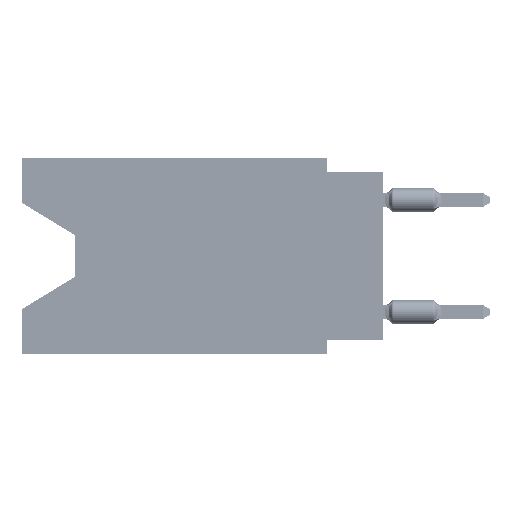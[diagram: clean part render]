
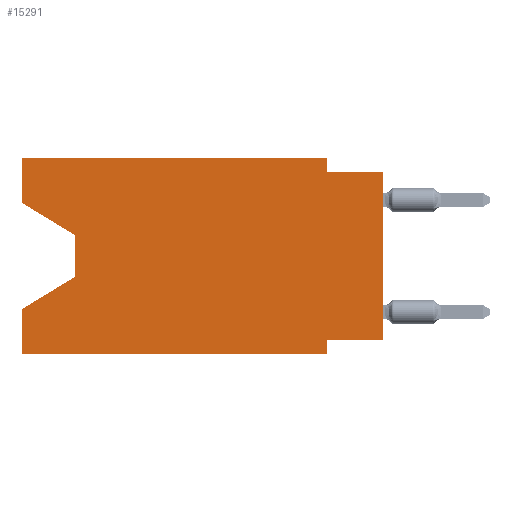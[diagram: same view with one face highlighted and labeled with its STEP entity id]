
A CAD part, left-side view. The second image highlights one B-rep face of the part: STEP entity #15291.
In plain terms, the highlighted planar face has unit normal (-1, 0, 0).
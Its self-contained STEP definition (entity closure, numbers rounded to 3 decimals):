
#107 = CARTESIAN_POINT ( 'NONE',  ( 0., 16.383, 0. ) ) ;
#763 = DIRECTION ( 'NONE',  ( 0., -0.855, -0.519 ) ) ;
#1878 = EDGE_CURVE ( 'NONE', #25673, #46017, #35333, .T. ) ;
#1930 = CARTESIAN_POINT ( 'NONE',  ( 0., 16.383, -2.038 ) ) ;
#2793 = AXIS2_PLACEMENT_3D ( 'NONE', #67931, #42210, #43051 ) ;
#2874 = DIRECTION ( 'NONE',  ( 0., 0., -1. ) ) ;
#2944 = VECTOR ( 'NONE', #48838, 1000. ) ;
#3037 = LINE ( 'NONE', #9887, #2944 ) ;
#4022 = LINE ( 'NONE', #82381, #73340 ) ;
#4577 = ORIENTED_EDGE ( 'NONE', *, *, #26708, .F. ) ;
#4982 = VECTOR ( 'NONE', #763, 1000. ) ;
#5463 = CARTESIAN_POINT ( 'NONE',  ( 0., 13.97, -5.385 ) ) ;
#9887 = CARTESIAN_POINT ( 'NONE',  ( 0., 16.383, 0. ) ) ;
#12253 = CARTESIAN_POINT ( 'NONE',  ( 0., 2.54, -8.255 ) ) ;
#14209 = LINE ( 'NONE', #107, #69110 ) ;
#15291 = ADVANCED_FACE ( 'NONE', ( #48216 ), #36222, .F. ) ;
#15348 = EDGE_CURVE ( 'NONE', #16170, #65032, #21712, .T. ) ;
#16145 = LINE ( 'NONE', #35400, #50735 ) ;
#16170 = VERTEX_POINT ( 'NONE', #39067 ) ;
#16558 = DIRECTION ( 'NONE',  ( 0., -1., 0. ) ) ;
#16648 = VECTOR ( 'NONE', #29829, 1000. ) ;
#17340 = EDGE_CURVE ( 'NONE', #54386, #83672, #40953, .T. ) ;
#19765 = EDGE_CURVE ( 'NONE', #46017, #43239, #67621, .T. ) ;
#20991 = CARTESIAN_POINT ( 'NONE',  ( 0., 16.383, -8.89 ) ) ;
#21712 = LINE ( 'NONE', #22974, #43765 ) ;
#22974 = CARTESIAN_POINT ( 'NONE',  ( 0., 0., -8.255 ) ) ;
#23085 = CARTESIAN_POINT ( 'NONE',  ( 0., 0., -0.635 ) ) ;
#23415 = CARTESIAN_POINT ( 'NONE',  ( 0., 13.97, -3.505 ) ) ;
#25673 = VERTEX_POINT ( 'NONE', #26415 ) ;
#26223 = CARTESIAN_POINT ( 'NONE',  ( 0., 0., 0. ) ) ;
#26322 = VECTOR ( 'NONE', #49864, 1000. ) ;
#26415 = CARTESIAN_POINT ( 'NONE',  ( 0., 2.54, 0. ) ) ;
#26708 = EDGE_CURVE ( 'NONE', #51385, #32108, #3037, .T. ) ;
#26897 = EDGE_CURVE ( 'NONE', #65584, #54386, #36257, .T. ) ;
#27863 = CARTESIAN_POINT ( 'NONE',  ( 0., 16.383, -6.852 ) ) ;
#28916 = CARTESIAN_POINT ( 'NONE',  ( 0., 2.54, 0. ) ) ;
#29567 = ORIENTED_EDGE ( 'NONE', *, *, #56572, .T. ) ;
#29829 = DIRECTION ( 'NONE',  ( 0., 0.855, -0.519 ) ) ;
#30577 = CARTESIAN_POINT ( 'NONE',  ( 0., 2.54, -0.635 ) ) ;
#30886 = CARTESIAN_POINT ( 'NONE',  ( 0., 16.383, 0. ) ) ;
#32008 = ORIENTED_EDGE ( 'NONE', *, *, #26897, .T. ) ;
#32108 = VERTEX_POINT ( 'NONE', #30886 ) ;
#33012 = EDGE_CURVE ( 'NONE', #51385, #65584, #46971, .T. ) ;
#34096 = ORIENTED_EDGE ( 'NONE', *, *, #78147, .F. ) ;
#35333 = LINE ( 'NONE', #28916, #26322 ) ;
#35400 = CARTESIAN_POINT ( 'NONE',  ( 0., 16.383, 0. ) ) ;
#35809 = CARTESIAN_POINT ( 'NONE',  ( 0., 13.97, -5.385 ) ) ;
#36135 = DIRECTION ( 'NONE',  ( 0., 0., -1. ) ) ;
#36222 = PLANE ( 'NONE',  #2793 ) ;
#36257 = LINE ( 'NONE', #23415, #58999 ) ;
#37392 = CARTESIAN_POINT ( 'NONE',  ( 0., 2.54, -8.89 ) ) ;
#37627 = ORIENTED_EDGE ( 'NONE', *, *, #15348, .F. ) ;
#38534 = CARTESIAN_POINT ( 'NONE',  ( 0., 16.383, -8.89 ) ) ;
#38618 = LINE ( 'NONE', #26223, #69761 ) ;
#38981 = EDGE_CURVE ( 'NONE', #76979, #78076, #71090, .T. ) ;
#39067 = CARTESIAN_POINT ( 'NONE',  ( 0., 0., -8.255 ) ) ;
#40325 = DIRECTION ( 'NONE',  ( 0., 0., 1. ) ) ;
#40589 = ORIENTED_EDGE ( 'NONE', *, *, #38981, .T. ) ;
#40953 = LINE ( 'NONE', #35809, #16648 ) ;
#42210 = DIRECTION ( 'NONE',  ( 1., 0., 0. ) ) ;
#43051 = DIRECTION ( 'NONE',  ( 0., 0., -1. ) ) ;
#43239 = VERTEX_POINT ( 'NONE', #73313 ) ;
#43765 = VECTOR ( 'NONE', #68768, 1000. ) ;
#45612 = EDGE_CURVE ( 'NONE', #32108, #25673, #16145, .T. ) ;
#45690 = VECTOR ( 'NONE', #75317, 1000. ) ;
#46017 = VERTEX_POINT ( 'NONE', #30577 ) ;
#46971 = LINE ( 'NONE', #73101, #4982 ) ;
#47459 = VECTOR ( 'NONE', #57401, 1000. ) ;
#48216 = FACE_OUTER_BOUND ( 'NONE', #61490, .T. ) ;
#48838 = DIRECTION ( 'NONE',  ( 0., 0., 1. ) ) ;
#49864 = DIRECTION ( 'NONE',  ( 0., 0., -1. ) ) ;
#50735 = VECTOR ( 'NONE', #16558, 1000. ) ;
#51385 = VERTEX_POINT ( 'NONE', #1930 ) ;
#54386 = VERTEX_POINT ( 'NONE', #5463 ) ;
#54658 = ORIENTED_EDGE ( 'NONE', *, *, #33012, .T. ) ;
#56572 = EDGE_CURVE ( 'NONE', #16170, #43239, #38618, .T. ) ;
#57401 = DIRECTION ( 'NONE',  ( 0., -1., 0. ) ) ;
#58999 = VECTOR ( 'NONE', #2874, 1000. ) ;
#61490 = EDGE_LOOP ( 'NONE', ( #54658, #32008, #80847, #71465, #40589, #34096, #37627, #29567, #69365, #63254, #64723, #4577 ) ) ;
#62638 = EDGE_CURVE ( 'NONE', #76979, #83672, #14209, .T. ) ;
#63254 = ORIENTED_EDGE ( 'NONE', *, *, #1878, .F. ) ;
#64723 = ORIENTED_EDGE ( 'NONE', *, *, #45612, .F. ) ;
#65032 = VERTEX_POINT ( 'NONE', #12253 ) ;
#65584 = VERTEX_POINT ( 'NONE', #72973 ) ;
#67621 = LINE ( 'NONE', #23085, #45690 ) ;
#67931 = CARTESIAN_POINT ( 'NONE',  ( 0., 16.383, 0. ) ) ;
#68768 = DIRECTION ( 'NONE',  ( 0., 1., 0. ) ) ;
#69110 = VECTOR ( 'NONE', #40325, 1000. ) ;
#69365 = ORIENTED_EDGE ( 'NONE', *, *, #19765, .F. ) ;
#69761 = VECTOR ( 'NONE', #84040, 1000. ) ;
#71090 = LINE ( 'NONE', #38534, #47459 ) ;
#71465 = ORIENTED_EDGE ( 'NONE', *, *, #62638, .F. ) ;
#72973 = CARTESIAN_POINT ( 'NONE',  ( 0., 13.97, -3.505 ) ) ;
#73101 = CARTESIAN_POINT ( 'NONE',  ( 0., 16.383, -2.038 ) ) ;
#73313 = CARTESIAN_POINT ( 'NONE',  ( 0., 0., -0.635 ) ) ;
#73340 = VECTOR ( 'NONE', #36135, 1000. ) ;
#75317 = DIRECTION ( 'NONE',  ( 0., -1., 0. ) ) ;
#76979 = VERTEX_POINT ( 'NONE', #20991 ) ;
#78076 = VERTEX_POINT ( 'NONE', #37392 ) ;
#78147 = EDGE_CURVE ( 'NONE', #65032, #78076, #4022, .T. ) ;
#80847 = ORIENTED_EDGE ( 'NONE', *, *, #17340, .T. ) ;
#82381 = CARTESIAN_POINT ( 'NONE',  ( 0., 2.54, -8.89 ) ) ;
#83672 = VERTEX_POINT ( 'NONE', #27863 ) ;
#84040 = DIRECTION ( 'NONE',  ( 0., 0., 1. ) ) ;
